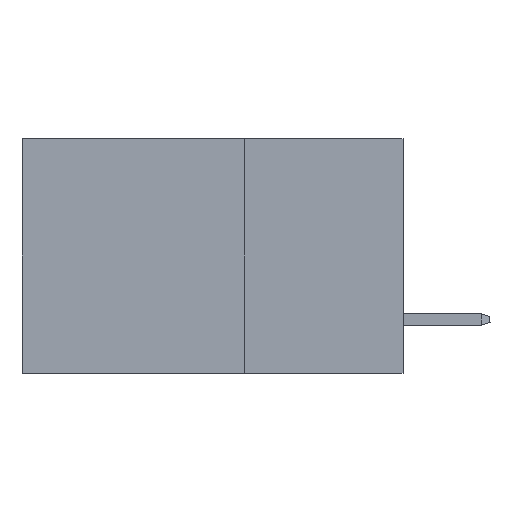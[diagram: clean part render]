
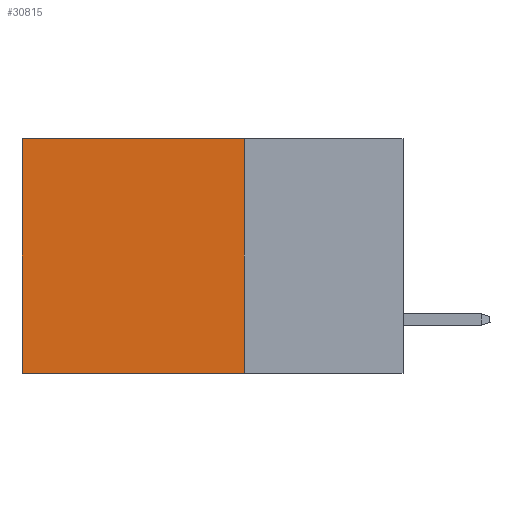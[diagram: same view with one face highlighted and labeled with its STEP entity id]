
A CAD part, left-side view. The second image highlights one B-rep face of the part: STEP entity #30815.
In plain terms, the highlighted planar face has unit normal (-1, 0, 0).
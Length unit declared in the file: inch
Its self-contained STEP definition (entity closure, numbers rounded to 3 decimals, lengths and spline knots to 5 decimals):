
#601 = CARTESIAN_POINT ( 'NONE',  ( 0.2875, 0.25, 0. ) ) ;
#1307 = EDGE_CURVE ( 'NONE', #23105, #25768, #16199, .T. ) ;
#1874 = LINE ( 'NONE', #3863, #19370 ) ;
#2749 = LINE ( 'NONE', #601, #4527 ) ;
#3863 = CARTESIAN_POINT ( 'NONE',  ( 0.2875, 0.6, 0. ) ) ;
#4527 = VECTOR ( 'NONE', #16689, 39.37008 ) ;
#9152 = EDGE_CURVE ( 'NONE', #23105, #11621, #2749, .T. ) ;
#10097 = EDGE_CURVE ( 'NONE', #11621, #29821, #1874, .T. ) ;
#10636 = CARTESIAN_POINT ( 'NONE',  ( 0.2875, 0.25, -0.37 ) ) ;
#11621 = VERTEX_POINT ( 'NONE', #35016 ) ;
#11740 = FACE_OUTER_BOUND ( 'NONE', #22458, .T. ) ;
#16199 = LINE ( 'NONE', #35227, #22768 ) ;
#16689 = DIRECTION ( 'NONE',  ( 0., 1., 0. ) ) ;
#17056 = ORIENTED_EDGE ( 'NONE', *, *, #21706, .F. ) ;
#17877 = ORIENTED_EDGE ( 'NONE', *, *, #10097, .T. ) ;
#18145 = DIRECTION ( 'NONE',  ( 0., 0., -1. ) ) ;
#19370 = VECTOR ( 'NONE', #18145, 39.37008 ) ;
#19991 = DIRECTION ( 'NONE',  ( 0., 0., -1. ) ) ;
#21706 = EDGE_CURVE ( 'NONE', #25768, #29821, #21781, .T. ) ;
#21781 = LINE ( 'NONE', #33075, #31331 ) ;
#22111 = DIRECTION ( 'NONE',  ( 0., 0., -1. ) ) ;
#22458 = EDGE_LOOP ( 'NONE', ( #17877, #17056, #34084, #30669 ) ) ;
#22572 = CARTESIAN_POINT ( 'NONE',  ( 0.2875, 0.6, -0.37 ) ) ;
#22768 = VECTOR ( 'NONE', #22111, 39.37008 ) ;
#23105 = VERTEX_POINT ( 'NONE', #27561 ) ;
#25351 = DIRECTION ( 'NONE',  ( 1., 0., 0. ) ) ;
#25768 = VERTEX_POINT ( 'NONE', #10636 ) ;
#27492 = AXIS2_PLACEMENT_3D ( 'NONE', #31101, #25351, #19991 ) ;
#27561 = CARTESIAN_POINT ( 'NONE',  ( 0.2875, 0.25, 0. ) ) ;
#28748 = PLANE ( 'NONE',  #27492 ) ;
#29821 = VERTEX_POINT ( 'NONE', #22572 ) ;
#30669 = ORIENTED_EDGE ( 'NONE', *, *, #9152, .T. ) ;
#30815 = ADVANCED_FACE ( 'NONE', ( #11740 ), #28748, .F. ) ;
#31101 = CARTESIAN_POINT ( 'NONE',  ( 0.2875, 0.25, 0. ) ) ;
#31331 = VECTOR ( 'NONE', #33256, 39.37008 ) ;
#33075 = CARTESIAN_POINT ( 'NONE',  ( 0.2875, 0.25, -0.37 ) ) ;
#33256 = DIRECTION ( 'NONE',  ( 0., 1., 0. ) ) ;
#34084 = ORIENTED_EDGE ( 'NONE', *, *, #1307, .F. ) ;
#35016 = CARTESIAN_POINT ( 'NONE',  ( 0.2875, 0.6, 0. ) ) ;
#35227 = CARTESIAN_POINT ( 'NONE',  ( 0.2875, 0.25, 0. ) ) ;
